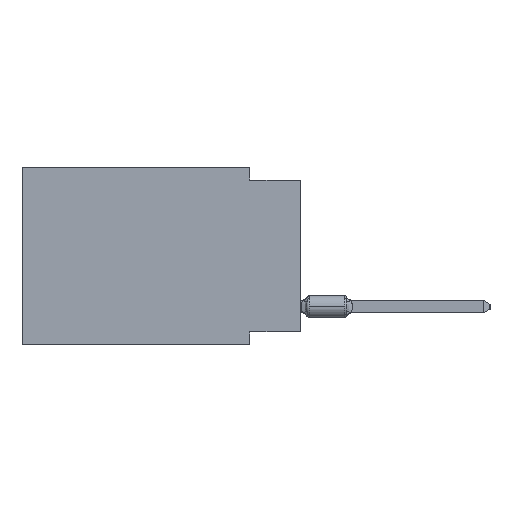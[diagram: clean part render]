
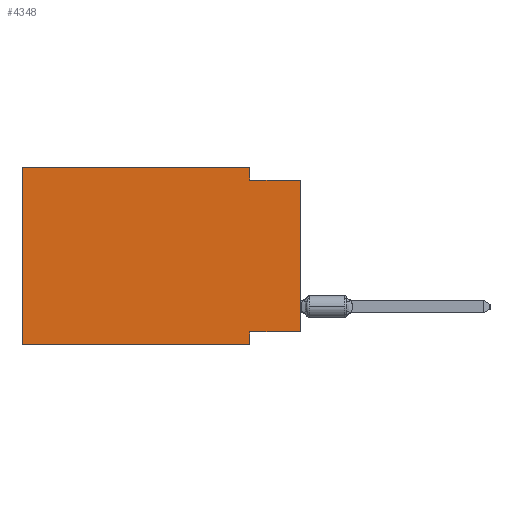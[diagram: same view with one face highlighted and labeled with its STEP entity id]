
A CAD part, left-side view. The second image highlights one B-rep face of the part: STEP entity #4348.
In plain terms, the highlighted planar face has unit normal (-1, 0, 0).
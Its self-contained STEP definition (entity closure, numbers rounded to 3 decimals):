
#1303 = DIRECTION ( 'NONE',  ( 1., 0., 0. ) ) ;
#1480 = LINE ( 'NONE', #42517, #18066 ) ;
#1641 = DIRECTION ( 'NONE',  ( 0., 0., -1. ) ) ;
#1961 = CARTESIAN_POINT ( 'NONE',  ( 0., 13.97, 0. ) ) ;
#4076 = ORIENTED_EDGE ( 'NONE', *, *, #32865, .T. ) ;
#4348 = ADVANCED_FACE ( 'NONE', ( #42023 ), #17283, .F. ) ;
#5183 = CARTESIAN_POINT ( 'NONE',  ( 0., 2.54, -8.255 ) ) ;
#6813 = DIRECTION ( 'NONE',  ( 0., -1., 0. ) ) ;
#7522 = CARTESIAN_POINT ( 'NONE',  ( 0., 2.54, -8.89 ) ) ;
#8870 = DIRECTION ( 'NONE',  ( 0., 0., -1. ) ) ;
#8913 = VERTEX_POINT ( 'NONE', #7522 ) ;
#9003 = VERTEX_POINT ( 'NONE', #50204 ) ;
#9949 = LINE ( 'NONE', #50331, #27546 ) ;
#11398 = EDGE_CURVE ( 'NONE', #34783, #8913, #17438, .T. ) ;
#12086 = CARTESIAN_POINT ( 'NONE',  ( 0., 0., -8.255 ) ) ;
#12836 = VECTOR ( 'NONE', #15679, 1000. ) ;
#14138 = LINE ( 'NONE', #53826, #55717 ) ;
#14609 = DIRECTION ( 'NONE',  ( 0., 0., 1. ) ) ;
#15414 = DIRECTION ( 'NONE',  ( 0., 0., 1. ) ) ;
#15679 = DIRECTION ( 'NONE',  ( 0., -1., 0. ) ) ;
#17283 = PLANE ( 'NONE',  #50566 ) ;
#17365 = VERTEX_POINT ( 'NONE', #65400 ) ;
#17438 = LINE ( 'NONE', #53155, #44696 ) ;
#18066 = VECTOR ( 'NONE', #6813, 1000. ) ;
#18725 = LINE ( 'NONE', #55115, #49426 ) ;
#19592 = CARTESIAN_POINT ( 'NONE',  ( 0., 13.97, -8.89 ) ) ;
#20672 = EDGE_CURVE ( 'NONE', #9003, #63789, #60934, .T. ) ;
#22009 = VERTEX_POINT ( 'NONE', #12086 ) ;
#24590 = ORIENTED_EDGE ( 'NONE', *, *, #62685, .F. ) ;
#25201 = CARTESIAN_POINT ( 'NONE',  ( 0., 2.54, 0. ) ) ;
#25738 = CARTESIAN_POINT ( 'NONE',  ( 0., 13.97, 0. ) ) ;
#25960 = EDGE_CURVE ( 'NONE', #22009, #17365, #9949, .T. ) ;
#26909 = VECTOR ( 'NONE', #15414, 1000. ) ;
#27546 = VECTOR ( 'NONE', #14609, 1000. ) ;
#28583 = ORIENTED_EDGE ( 'NONE', *, *, #25960, .T. ) ;
#30060 = DIRECTION ( 'NONE',  ( 0., 1., 0. ) ) ;
#30165 = ORIENTED_EDGE ( 'NONE', *, *, #62909, .F. ) ;
#32865 = EDGE_CURVE ( 'NONE', #64963, #8913, #60770, .T. ) ;
#34445 = DIRECTION ( 'NONE',  ( 0., -1., 0. ) ) ;
#34740 = CARTESIAN_POINT ( 'NONE',  ( 0., 13.97, -8.89 ) ) ;
#34783 = VERTEX_POINT ( 'NONE', #5183 ) ;
#37954 = ORIENTED_EDGE ( 'NONE', *, *, #40833, .F. ) ;
#38328 = ORIENTED_EDGE ( 'NONE', *, *, #46807, .F. ) ;
#40833 = EDGE_CURVE ( 'NONE', #64510, #9003, #1480, .T. ) ;
#42023 = FACE_OUTER_BOUND ( 'NONE', #51808, .T. ) ;
#42517 = CARTESIAN_POINT ( 'NONE',  ( 0., 13.97, 0. ) ) ;
#44696 = VECTOR ( 'NONE', #49059, 1000. ) ;
#46292 = CARTESIAN_POINT ( 'NONE',  ( 0., 2.54, -0.635 ) ) ;
#46807 = EDGE_CURVE ( 'NONE', #22009, #34783, #18725, .T. ) ;
#47668 = ORIENTED_EDGE ( 'NONE', *, *, #20672, .F. ) ;
#49059 = DIRECTION ( 'NONE',  ( 0., 0., -1. ) ) ;
#49426 = VECTOR ( 'NONE', #30060, 1000. ) ;
#50204 = CARTESIAN_POINT ( 'NONE',  ( 0., 2.54, 0. ) ) ;
#50331 = CARTESIAN_POINT ( 'NONE',  ( 0., 0., 0. ) ) ;
#50566 = AXIS2_PLACEMENT_3D ( 'NONE', #1961, #1303, #1641 ) ;
#51808 = EDGE_LOOP ( 'NONE', ( #28583, #24590, #47668, #37954, #30165, #4076, #52589, #38328 ) ) ;
#52589 = ORIENTED_EDGE ( 'NONE', *, *, #11398, .F. ) ;
#53155 = CARTESIAN_POINT ( 'NONE',  ( 0., 2.54, -8.89 ) ) ;
#53826 = CARTESIAN_POINT ( 'NONE',  ( 0., 0., -0.635 ) ) ;
#55115 = CARTESIAN_POINT ( 'NONE',  ( 0., 0., -8.255 ) ) ;
#55717 = VECTOR ( 'NONE', #34445, 1000. ) ;
#56731 = CARTESIAN_POINT ( 'NONE',  ( 0., 13.97, 0. ) ) ;
#60770 = LINE ( 'NONE', #34740, #12836 ) ;
#60934 = LINE ( 'NONE', #25201, #62189 ) ;
#61151 = LINE ( 'NONE', #25738, #26909 ) ;
#62189 = VECTOR ( 'NONE', #8870, 1000. ) ;
#62685 = EDGE_CURVE ( 'NONE', #63789, #17365, #14138, .T. ) ;
#62909 = EDGE_CURVE ( 'NONE', #64963, #64510, #61151, .T. ) ;
#63789 = VERTEX_POINT ( 'NONE', #46292 ) ;
#64510 = VERTEX_POINT ( 'NONE', #56731 ) ;
#64963 = VERTEX_POINT ( 'NONE', #19592 ) ;
#65400 = CARTESIAN_POINT ( 'NONE',  ( 0., 0., -0.635 ) ) ;
